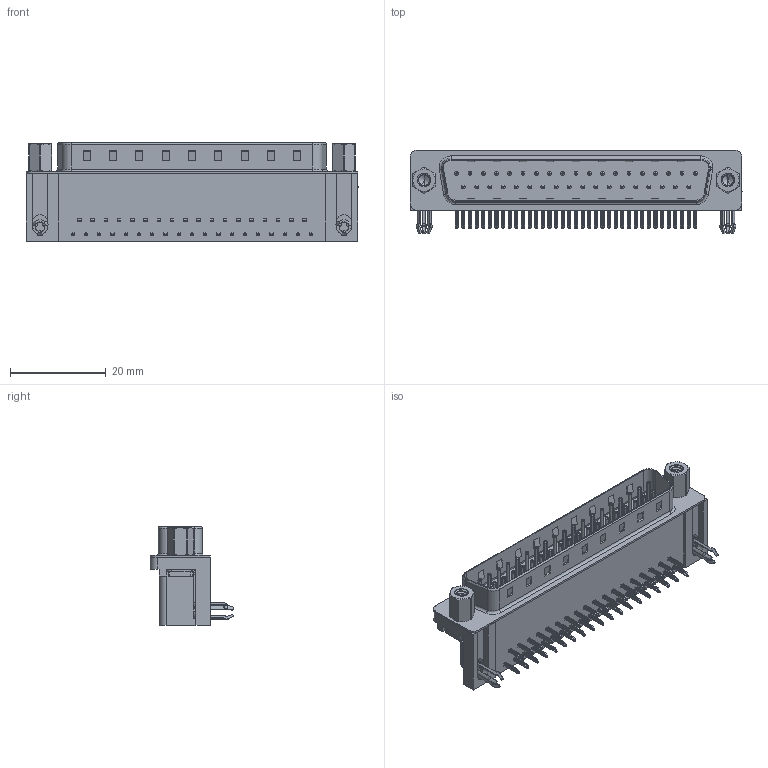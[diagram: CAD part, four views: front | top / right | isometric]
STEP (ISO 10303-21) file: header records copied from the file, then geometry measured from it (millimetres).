
FILE_DESCRIPTION (( 'STEP AP203' ), '1' );
FILE_NAME ('629-037-340-043.STEP', '2021-09-21T20:59:24', ( '' ), ( '' ), 'SwSTEP 2.0', 'SolidWorks 2020', '' );
FILE_SCHEMA (( 'CONFIG_CONTROL_DESIGN' ));
Length unit declared in the file: millimetre
Products named in the file (8): 629 4-40 Hex Standoff 5; 629 Shell_37 Socket; 629 3 Prong Board Lock; 629 Housing_37 Socket; 629-037-340-043; 629 4-40 Threaded Rivet; 629 Contact Top; 629 Contact Bottom
Assembly tree (45 placements, depth 2):
  629-037-340-043
    629 Housing_37 Socket
    629 Shell_37 Socket
    629 Contact Bottom  x18
    629 Contact Top  x19
    629 3 Prong Board Lock  x2
    629 4-40 Threaded Rivet  x2
    629 4-40 Hex Standoff 5  x2
Bounding box: 69.4 x 17.48 x 20.6 mm (x, y, z)
Volume: 10191.6 mm3; surface area: 11368.8 mm2
Topology: 45 solids, 45 shells, 3427 faces, 8555 edges, 5299 vertices
Faces by surface type: plane 2071, cylinder 993, torus 277, cone 68, bspline 18
Entity records: 33298 total; most frequent: CARTESIAN_POINT 9373, DIRECTION 4609, ORIENTED_EDGE 4542, EDGE_CURVE 2271, LINE 1539, VECTOR 1539, AXIS2_PLACEMENT_3D 1535, VERTEX_POINT 1468
